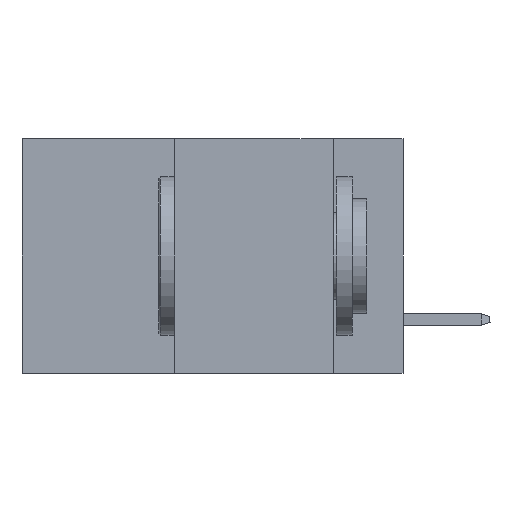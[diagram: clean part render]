
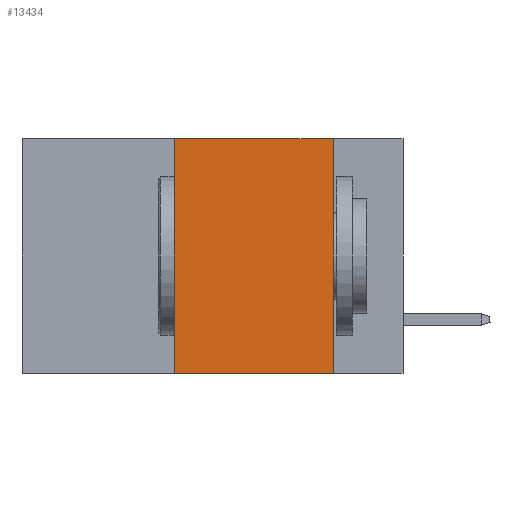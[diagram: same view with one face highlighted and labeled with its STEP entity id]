
A CAD part, left-side view. The second image highlights one B-rep face of the part: STEP entity #13434.
In plain terms, the highlighted planar face has unit normal (-1, 0, 0).
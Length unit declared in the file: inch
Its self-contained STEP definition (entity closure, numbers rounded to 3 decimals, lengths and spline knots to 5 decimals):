
#338 = VECTOR ( 'NONE', #3268, 39.37008 ) ;
#1329 = ORIENTED_EDGE ( 'NONE', *, *, #6914, .F. ) ;
#1409 = PLANE ( 'NONE',  #16694 ) ;
#1436 = CARTESIAN_POINT ( 'NONE',  ( 0., 0.36, -0.37 ) ) ;
#3268 = DIRECTION ( 'NONE',  ( 0., 0., 1. ) ) ;
#5156 = ORIENTED_EDGE ( 'NONE', *, *, #5579, .F. ) ;
#5579 = EDGE_CURVE ( 'NONE', #7303, #11229, #19551, .T. ) ;
#6914 = EDGE_CURVE ( 'NONE', #18378, #7303, #13068, .T. ) ;
#7303 = VERTEX_POINT ( 'NONE', #16873 ) ;
#7424 = DIRECTION ( 'NONE',  ( 0., 0., -1. ) ) ;
#7937 = EDGE_CURVE ( 'NONE', #18378, #9238, #10416, .T. ) ;
#8145 = EDGE_LOOP ( 'NONE', ( #15186, #5156, #1329, #11671 ) ) ;
#8801 = CARTESIAN_POINT ( 'NONE',  ( 0., 0.6, 0. ) ) ;
#8833 = VECTOR ( 'NONE', #16895, 39.37008 ) ;
#9238 = VERTEX_POINT ( 'NONE', #11925 ) ;
#9500 = VECTOR ( 'NONE', #17463, 39.37008 ) ;
#9768 = CARTESIAN_POINT ( 'NONE',  ( 0., 0.6, -0.37 ) ) ;
#10416 = LINE ( 'NONE', #9768, #9500 ) ;
#11229 = VERTEX_POINT ( 'NONE', #11259 ) ;
#11259 = CARTESIAN_POINT ( 'NONE',  ( 0., 0.11, 0. ) ) ;
#11671 = ORIENTED_EDGE ( 'NONE', *, *, #7937, .T. ) ;
#11910 = DIRECTION ( 'NONE',  ( 0., 0., -1. ) ) ;
#11925 = CARTESIAN_POINT ( 'NONE',  ( 0., 0.11, -0.37 ) ) ;
#13068 = LINE ( 'NONE', #14474, #338 ) ;
#13434 = ADVANCED_FACE ( 'NONE', ( #15079 ), #1409, .F. ) ;
#13853 = CARTESIAN_POINT ( 'NONE',  ( 0., 0.6, 0. ) ) ;
#14474 = CARTESIAN_POINT ( 'NONE',  ( 0., 0.36, 0. ) ) ;
#15079 = FACE_OUTER_BOUND ( 'NONE', #8145, .T. ) ;
#15133 = LINE ( 'NONE', #18162, #16708 ) ;
#15186 = ORIENTED_EDGE ( 'NONE', *, *, #15487, .F. ) ;
#15487 = EDGE_CURVE ( 'NONE', #11229, #9238, #15133, .T. ) ;
#16694 = AXIS2_PLACEMENT_3D ( 'NONE', #13853, #18002, #11910 ) ;
#16708 = VECTOR ( 'NONE', #7424, 39.37008 ) ;
#16873 = CARTESIAN_POINT ( 'NONE',  ( 0., 0.36, 0. ) ) ;
#16895 = DIRECTION ( 'NONE',  ( 0., -1., 0. ) ) ;
#17463 = DIRECTION ( 'NONE',  ( 0., -1., 0. ) ) ;
#18002 = DIRECTION ( 'NONE',  ( 1., 0., 0. ) ) ;
#18162 = CARTESIAN_POINT ( 'NONE',  ( 0., 0.11, 0. ) ) ;
#18378 = VERTEX_POINT ( 'NONE', #1436 ) ;
#19551 = LINE ( 'NONE', #8801, #8833 ) ;
